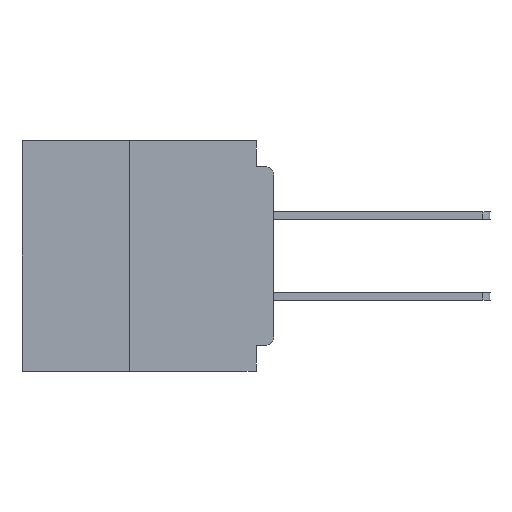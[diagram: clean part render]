
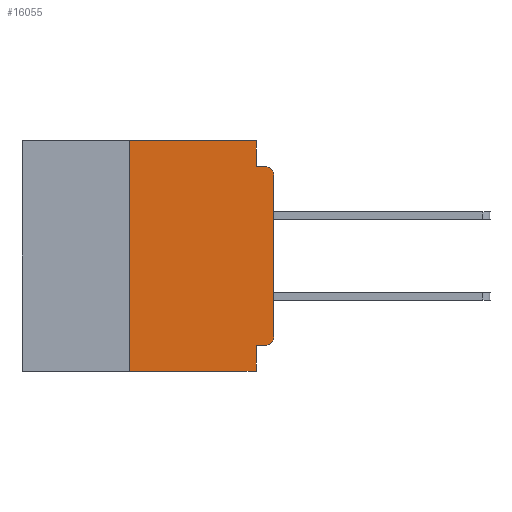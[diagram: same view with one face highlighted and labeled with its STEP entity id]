
A CAD part, left-side view. The second image highlights one B-rep face of the part: STEP entity #16055.
In plain terms, the highlighted planar face has unit normal (-1, 0, 0).
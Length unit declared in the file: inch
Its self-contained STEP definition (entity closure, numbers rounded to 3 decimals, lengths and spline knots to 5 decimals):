
#127 = DIRECTION ( 'NONE',  ( 0., -1., 0. ) ) ;
#315 = VECTOR ( 'NONE', #28744, 39.37008 ) ;
#1224 = DIRECTION ( 'NONE',  ( 0., 0., -1. ) ) ;
#2185 = LINE ( 'NONE', #16405, #47551 ) ;
#3406 = EDGE_CURVE ( 'NONE', #48896, #18432, #2185, .T. ) ;
#4242 = ORIENTED_EDGE ( 'NONE', *, *, #3406, .F. ) ;
#4366 = EDGE_CURVE ( 'NONE', #27255, #31040, #22599, .T. ) ;
#5888 = ORIENTED_EDGE ( 'NONE', *, *, #49532, .T. ) ;
#6047 = CARTESIAN_POINT ( 'NONE',  ( 0., 0., -0.34 ) ) ;
#6275 = FACE_OUTER_BOUND ( 'NONE', #8248, .T. ) ;
#7016 = DIRECTION ( 'NONE',  ( 0., 0., -1. ) ) ;
#7138 = VECTOR ( 'NONE', #57422, 39.37008 ) ;
#8248 = EDGE_LOOP ( 'NONE', ( #21046, #19652, #47978, #4242, #39174, #40024, #21661, #24484, #52840, #5888 ) ) ;
#9683 = DIRECTION ( 'NONE',  ( -1., 0., 0. ) ) ;
#9883 = CARTESIAN_POINT ( 'NONE',  ( 0., 0., -0.045 ) ) ;
#11539 = VERTEX_POINT ( 'NONE', #58357 ) ;
#12588 = CARTESIAN_POINT ( 'NONE',  ( 0., 0.031, -0.4 ) ) ;
#14227 = DIRECTION ( 'NONE',  ( 0., 0., 1. ) ) ;
#16055 = ADVANCED_FACE ( 'NONE', ( #6275 ), #52816, .F. ) ;
#16405 = CARTESIAN_POINT ( 'NONE',  ( 0., 0.031, 0. ) ) ;
#16631 = EDGE_CURVE ( 'NONE', #18432, #11539, #50059, .T. ) ;
#16660 = LINE ( 'NONE', #42295, #41575 ) ;
#17482 = AXIS2_PLACEMENT_3D ( 'NONE', #38760, #57486, #29617 ) ;
#18432 = VERTEX_POINT ( 'NONE', #37974 ) ;
#19652 = ORIENTED_EDGE ( 'NONE', *, *, #49414, .T. ) ;
#20524 = EDGE_CURVE ( 'NONE', #54861, #48896, #58401, .T. ) ;
#21046 = ORIENTED_EDGE ( 'NONE', *, *, #32282, .T. ) ;
#21172 = VECTOR ( 'NONE', #50423, 39.37008 ) ;
#21661 = ORIENTED_EDGE ( 'NONE', *, *, #4366, .T. ) ;
#22468 = CARTESIAN_POINT ( 'NONE',  ( 0., 0., -0.06 ) ) ;
#22599 = LINE ( 'NONE', #46779, #45985 ) ;
#24445 = AXIS2_PLACEMENT_3D ( 'NONE', #57224, #29341, #1224 ) ;
#24484 = ORIENTED_EDGE ( 'NONE', *, *, #42538, .F. ) ;
#24659 = CARTESIAN_POINT ( 'NONE',  ( 0., 0.25, -0.4 ) ) ;
#26800 = EDGE_CURVE ( 'NONE', #32293, #53923, #32757, .T. ) ;
#27255 = VERTEX_POINT ( 'NONE', #53103 ) ;
#27533 = VERTEX_POINT ( 'NONE', #22468 ) ;
#28744 = DIRECTION ( 'NONE',  ( 0., -1., 0. ) ) ;
#29341 = DIRECTION ( 'NONE',  ( -1., 0., 0. ) ) ;
#29617 = DIRECTION ( 'NONE',  ( 0., 0., -1. ) ) ;
#31040 = VERTEX_POINT ( 'NONE', #12588 ) ;
#31164 = CARTESIAN_POINT ( 'NONE',  ( 0., 0., -0.355 ) ) ;
#32282 = EDGE_CURVE ( 'NONE', #52670, #27533, #16660, .T. ) ;
#32293 = VERTEX_POINT ( 'NONE', #46948 ) ;
#32430 = EDGE_CURVE ( 'NONE', #27255, #54861, #48099, .T. ) ;
#32757 = LINE ( 'NONE', #31164, #43708 ) ;
#32998 = CIRCLE ( 'NONE', #50644, 0.015 ) ;
#34269 = VECTOR ( 'NONE', #57274, 39.37008 ) ;
#36323 = CARTESIAN_POINT ( 'NONE',  ( 0., 0.25, 0. ) ) ;
#36398 = CARTESIAN_POINT ( 'NONE',  ( 0., 0.437, 0. ) ) ;
#37713 = CARTESIAN_POINT ( 'NONE',  ( 0., 0.015, -0.06 ) ) ;
#37974 = CARTESIAN_POINT ( 'NONE',  ( 0., 0.031, -0.045 ) ) ;
#38691 = CARTESIAN_POINT ( 'NONE',  ( 0., 0.031, -0.4 ) ) ;
#38760 = CARTESIAN_POINT ( 'NONE',  ( 0., 0.437, 0. ) ) ;
#39174 = ORIENTED_EDGE ( 'NONE', *, *, #20524, .F. ) ;
#39867 = CARTESIAN_POINT ( 'NONE',  ( 0., 0.031, 0. ) ) ;
#40024 = ORIENTED_EDGE ( 'NONE', *, *, #32430, .F. ) ;
#40526 = DIRECTION ( 'NONE',  ( 0., 1., 0. ) ) ;
#41575 = VECTOR ( 'NONE', #14227, 39.37008 ) ;
#42295 = CARTESIAN_POINT ( 'NONE',  ( 0., 0., 0. ) ) ;
#42422 = DIRECTION ( 'NONE',  ( 0., 0., -1. ) ) ;
#42538 = EDGE_CURVE ( 'NONE', #53923, #31040, #44460, .T. ) ;
#43708 = VECTOR ( 'NONE', #40526, 39.37008 ) ;
#44460 = LINE ( 'NONE', #38691, #7138 ) ;
#45985 = VECTOR ( 'NONE', #127, 39.37008 ) ;
#46779 = CARTESIAN_POINT ( 'NONE',  ( 0., 0.437, -0.4 ) ) ;
#46948 = CARTESIAN_POINT ( 'NONE',  ( 0., 0.015, -0.355 ) ) ;
#47551 = VECTOR ( 'NONE', #7016, 39.37008 ) ;
#47978 = ORIENTED_EDGE ( 'NONE', *, *, #16631, .F. ) ;
#48099 = LINE ( 'NONE', #24659, #34269 ) ;
#48211 = CARTESIAN_POINT ( 'NONE',  ( 0., 0.031, -0.355 ) ) ;
#48896 = VERTEX_POINT ( 'NONE', #39867 ) ;
#49414 = EDGE_CURVE ( 'NONE', #27533, #11539, #32998, .T. ) ;
#49532 = EDGE_CURVE ( 'NONE', #32293, #52670, #50452, .T. ) ;
#50059 = LINE ( 'NONE', #9883, #315 ) ;
#50423 = DIRECTION ( 'NONE',  ( 0., -1., 0. ) ) ;
#50452 = CIRCLE ( 'NONE', #24445, 0.015 ) ;
#50644 = AXIS2_PLACEMENT_3D ( 'NONE', #37713, #9683, #42422 ) ;
#52670 = VERTEX_POINT ( 'NONE', #6047 ) ;
#52816 = PLANE ( 'NONE',  #17482 ) ;
#52840 = ORIENTED_EDGE ( 'NONE', *, *, #26800, .F. ) ;
#53103 = CARTESIAN_POINT ( 'NONE',  ( 0., 0.25, -0.4 ) ) ;
#53923 = VERTEX_POINT ( 'NONE', #48211 ) ;
#54861 = VERTEX_POINT ( 'NONE', #36323 ) ;
#57224 = CARTESIAN_POINT ( 'NONE',  ( 0., 0.015, -0.34 ) ) ;
#57274 = DIRECTION ( 'NONE',  ( 0., 0., 1. ) ) ;
#57422 = DIRECTION ( 'NONE',  ( 0., 0., -1. ) ) ;
#57486 = DIRECTION ( 'NONE',  ( 1., 0., 0. ) ) ;
#58357 = CARTESIAN_POINT ( 'NONE',  ( 0., 0.015, -0.045 ) ) ;
#58401 = LINE ( 'NONE', #36398, #21172 ) ;
